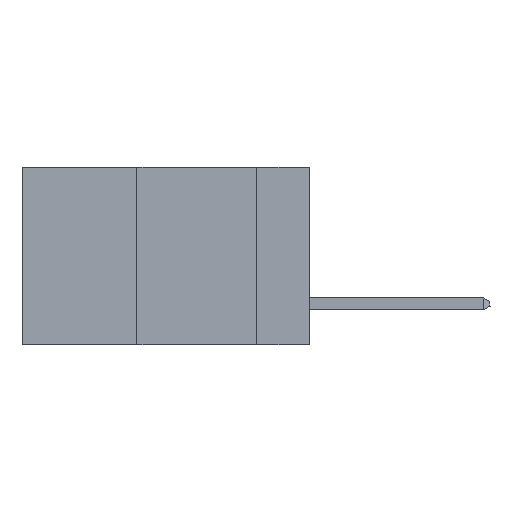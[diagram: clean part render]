
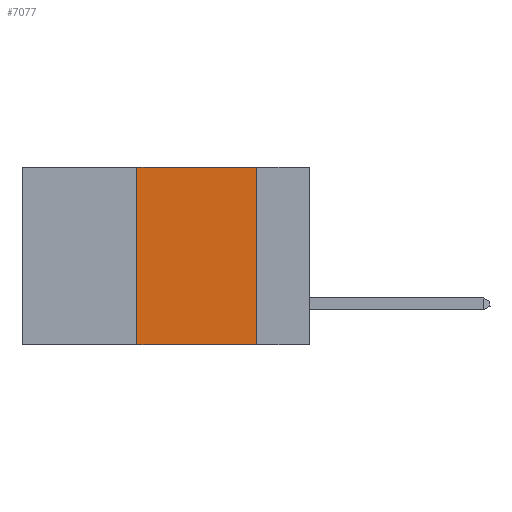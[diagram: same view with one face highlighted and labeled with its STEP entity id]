
A CAD part, left-side view. The second image highlights one B-rep face of the part: STEP entity #7077.
In plain terms, the highlighted planar face has unit normal (-1, 0, 0).
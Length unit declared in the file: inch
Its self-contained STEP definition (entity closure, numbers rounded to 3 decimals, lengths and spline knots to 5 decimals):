
#582 = VERTEX_POINT ( 'NONE', #1379 ) ;
#633 = DIRECTION ( 'NONE',  ( 0., 0., -1. ) ) ;
#1252 = EDGE_CURVE ( 'NONE', #9445, #6627, #1378, .T. ) ;
#1359 = ORIENTED_EDGE ( 'NONE', *, *, #3841, .F. ) ;
#1378 = LINE ( 'NONE', #9112, #1685 ) ;
#1379 = CARTESIAN_POINT ( 'NONE',  ( 0., 0.36, 0. ) ) ;
#1482 = DIRECTION ( 'NONE',  ( 1., 0., 0. ) ) ;
#1551 = EDGE_LOOP ( 'NONE', ( #2653, #1359, #5882, #7965 ) ) ;
#1685 = VECTOR ( 'NONE', #4439, 39.37008 ) ;
#1947 = LINE ( 'NONE', #3395, #6716 ) ;
#2505 = CARTESIAN_POINT ( 'NONE',  ( 0., 0.36, -0.37 ) ) ;
#2586 = DIRECTION ( 'NONE',  ( 0., -1., 0. ) ) ;
#2653 = ORIENTED_EDGE ( 'NONE', *, *, #1252, .F. ) ;
#2939 = LINE ( 'NONE', #8324, #8641 ) ;
#3395 = CARTESIAN_POINT ( 'NONE',  ( 0., 0.6, -0.37 ) ) ;
#3642 = CARTESIAN_POINT ( 'NONE',  ( 0., 0.6, 0. ) ) ;
#3653 = VECTOR ( 'NONE', #2586, 39.37008 ) ;
#3788 = PLANE ( 'NONE',  #6100 ) ;
#3841 = EDGE_CURVE ( 'NONE', #582, #9445, #5601, .T. ) ;
#4439 = DIRECTION ( 'NONE',  ( 0., 0., -1. ) ) ;
#4656 = CARTESIAN_POINT ( 'NONE',  ( 0., 0.11, -0.37 ) ) ;
#4986 = EDGE_CURVE ( 'NONE', #6396, #6627, #1947, .T. ) ;
#5110 = DIRECTION ( 'NONE',  ( 0., -1., 0. ) ) ;
#5601 = LINE ( 'NONE', #8611, #3653 ) ;
#5722 = EDGE_CURVE ( 'NONE', #6396, #582, #2939, .T. ) ;
#5882 = ORIENTED_EDGE ( 'NONE', *, *, #5722, .F. ) ;
#6042 = CARTESIAN_POINT ( 'NONE',  ( 0., 0.11, 0. ) ) ;
#6058 = DIRECTION ( 'NONE',  ( 0., 0., 1. ) ) ;
#6100 = AXIS2_PLACEMENT_3D ( 'NONE', #3642, #1482, #633 ) ;
#6396 = VERTEX_POINT ( 'NONE', #2505 ) ;
#6627 = VERTEX_POINT ( 'NONE', #4656 ) ;
#6716 = VECTOR ( 'NONE', #5110, 39.37008 ) ;
#7077 = ADVANCED_FACE ( 'NONE', ( #9069 ), #3788, .F. ) ;
#7965 = ORIENTED_EDGE ( 'NONE', *, *, #4986, .T. ) ;
#8324 = CARTESIAN_POINT ( 'NONE',  ( 0., 0.36, 0. ) ) ;
#8611 = CARTESIAN_POINT ( 'NONE',  ( 0., 0.6, 0. ) ) ;
#8641 = VECTOR ( 'NONE', #6058, 39.37008 ) ;
#9069 = FACE_OUTER_BOUND ( 'NONE', #1551, .T. ) ;
#9112 = CARTESIAN_POINT ( 'NONE',  ( 0., 0.11, 0. ) ) ;
#9445 = VERTEX_POINT ( 'NONE', #6042 ) ;
